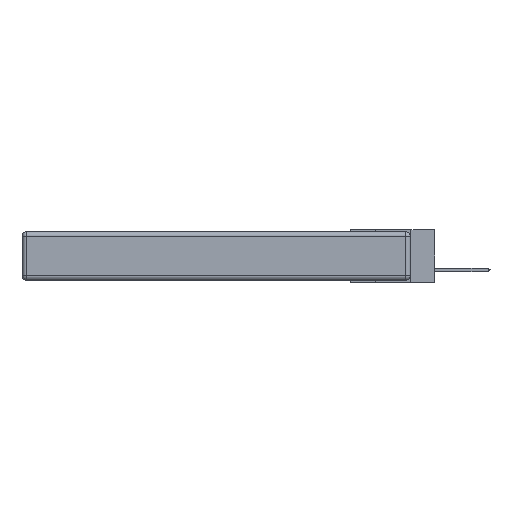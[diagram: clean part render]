
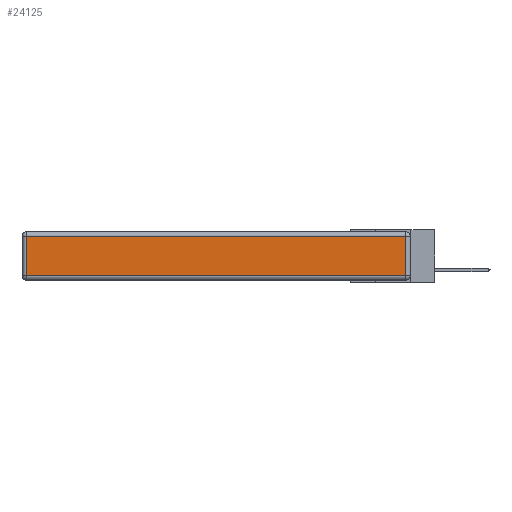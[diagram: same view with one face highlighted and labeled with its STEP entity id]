
A CAD part, left-side view. The second image highlights one B-rep face of the part: STEP entity #24125.
In plain terms, the highlighted planar face has unit normal (-1, 0, 0).
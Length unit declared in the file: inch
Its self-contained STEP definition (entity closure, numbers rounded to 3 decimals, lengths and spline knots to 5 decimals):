
#2277 = ORIENTED_EDGE ( 'NONE', *, *, #11956, .T. ) ;
#2576 = VERTEX_POINT ( 'NONE', #7926 ) ;
#3247 = ORIENTED_EDGE ( 'NONE', *, *, #14730, .T. ) ;
#4356 = DIRECTION ( 'NONE',  ( 0., 0., 1. ) ) ;
#4828 = PLANE ( 'NONE',  #13329 ) ;
#4834 = LINE ( 'NONE', #12376, #25662 ) ;
#5342 = LINE ( 'NONE', #14278, #21745 ) ;
#6187 = ORIENTED_EDGE ( 'NONE', *, *, #21578, .T. ) ;
#7540 = CARTESIAN_POINT ( 'NONE',  ( 0., 2.75, -0.03 ) ) ;
#7926 = CARTESIAN_POINT ( 'NONE',  ( 0., 0.03, -0.03 ) ) ;
#8112 = DIRECTION ( 'NONE',  ( 0., -1., 0. ) ) ;
#8271 = CARTESIAN_POINT ( 'NONE',  ( 0., 2.72, -0.03 ) ) ;
#9083 = VECTOR ( 'NONE', #4356, 39.37008 ) ;
#9485 = DIRECTION ( 'NONE',  ( 0., 0., -1. ) ) ;
#10356 = VERTEX_POINT ( 'NONE', #8271 ) ;
#11522 = CARTESIAN_POINT ( 'NONE',  ( 0., 2.72, -0.313 ) ) ;
#11956 = EDGE_CURVE ( 'NONE', #18197, #2576, #19798, .T. ) ;
#12376 = CARTESIAN_POINT ( 'NONE',  ( 0., 2.72, -0.343 ) ) ;
#12461 = ORIENTED_EDGE ( 'NONE', *, *, #23639, .T. ) ;
#13329 = AXIS2_PLACEMENT_3D ( 'NONE', #19200, #19018, #25200 ) ;
#14278 = CARTESIAN_POINT ( 'NONE',  ( 0., 0., -0.313 ) ) ;
#14730 = EDGE_CURVE ( 'NONE', #10356, #18165, #4834, .T. ) ;
#15799 = EDGE_LOOP ( 'NONE', ( #12461, #2277, #6187, #3247 ) ) ;
#16713 = CARTESIAN_POINT ( 'NONE',  ( 0., 0.03, -0.343 ) ) ;
#17696 = DIRECTION ( 'NONE',  ( 0., 1., 0. ) ) ;
#17758 = LINE ( 'NONE', #7540, #22495 ) ;
#18165 = VERTEX_POINT ( 'NONE', #11522 ) ;
#18197 = VERTEX_POINT ( 'NONE', #20187 ) ;
#19018 = DIRECTION ( 'NONE',  ( -1., 0., 0. ) ) ;
#19200 = CARTESIAN_POINT ( 'NONE',  ( 0., 0., -0.343 ) ) ;
#19798 = LINE ( 'NONE', #16713, #9083 ) ;
#20187 = CARTESIAN_POINT ( 'NONE',  ( 0., 0.03, -0.313 ) ) ;
#21578 = EDGE_CURVE ( 'NONE', #2576, #10356, #17758, .T. ) ;
#21745 = VECTOR ( 'NONE', #8112, 39.37008 ) ;
#22495 = VECTOR ( 'NONE', #17696, 39.37008 ) ;
#23639 = EDGE_CURVE ( 'NONE', #18165, #18197, #5342, .T. ) ;
#24125 = ADVANCED_FACE ( 'NONE', ( #25510 ), #4828, .T. ) ;
#25200 = DIRECTION ( 'NONE',  ( 0., 0., 1. ) ) ;
#25510 = FACE_OUTER_BOUND ( 'NONE', #15799, .T. ) ;
#25662 = VECTOR ( 'NONE', #9485, 39.37008 ) ;
